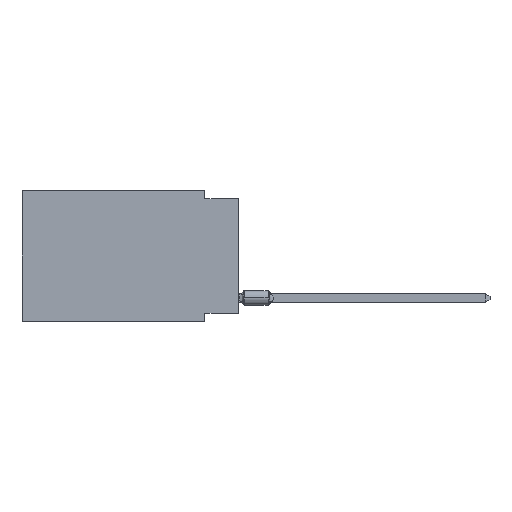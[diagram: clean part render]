
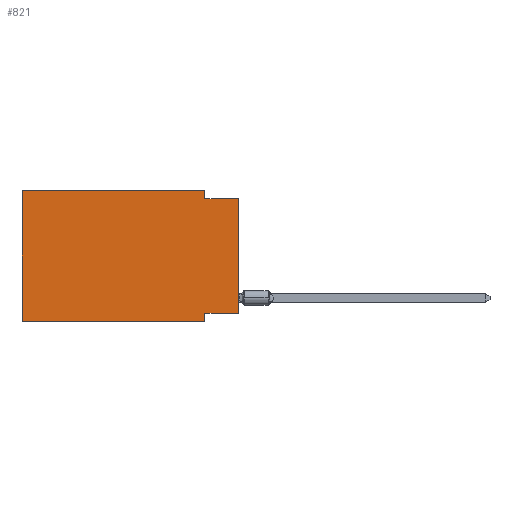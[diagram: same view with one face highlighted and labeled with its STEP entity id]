
A CAD part, left-side view. The second image highlights one B-rep face of the part: STEP entity #821.
In plain terms, the highlighted planar face has unit normal (-1, 0, 0).
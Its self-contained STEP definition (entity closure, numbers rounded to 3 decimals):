
#77 = VECTOR ( 'NONE', #10735, 1000. ) ;
#146 = DIRECTION ( 'NONE',  ( 0., 1., 0. ) ) ;
#390 = CARTESIAN_POINT ( 'NONE',  ( 0., 16.383, 0. ) ) ;
#655 = ORIENTED_EDGE ( 'NONE', *, *, #11525, .T. ) ;
#775 = CARTESIAN_POINT ( 'NONE',  ( 0., 2.54, 0. ) ) ;
#782 = FACE_OUTER_BOUND ( 'NONE', #11068, .T. ) ;
#821 = ADVANCED_FACE ( 'NONE', ( #782 ), #12748, .F. ) ;
#913 = DIRECTION ( 'NONE',  ( 1., 0., 0. ) ) ;
#946 = ORIENTED_EDGE ( 'NONE', *, *, #5960, .F. ) ;
#1041 = DIRECTION ( 'NONE',  ( 0., 0., -1. ) ) ;
#1175 = CARTESIAN_POINT ( 'NONE',  ( 0., 0., -0.635 ) ) ;
#1283 = EDGE_CURVE ( 'NONE', #8576, #7658, #7881, .T. ) ;
#1309 = CARTESIAN_POINT ( 'NONE',  ( 0., 0., -9.271 ) ) ;
#1402 = VECTOR ( 'NONE', #9608, 1000. ) ;
#2330 = CARTESIAN_POINT ( 'NONE',  ( 0., 16.383, -9.906 ) ) ;
#2385 = VECTOR ( 'NONE', #2811, 1000. ) ;
#2516 = VERTEX_POINT ( 'NONE', #5256 ) ;
#2692 = LINE ( 'NONE', #8646, #1402 ) ;
#2745 = CARTESIAN_POINT ( 'NONE',  ( 0., 16.383, 0. ) ) ;
#2811 = DIRECTION ( 'NONE',  ( 0., 0., 1. ) ) ;
#3001 = VECTOR ( 'NONE', #12733, 1000. ) ;
#3041 = ORIENTED_EDGE ( 'NONE', *, *, #8999, .F. ) ;
#3194 = DIRECTION ( 'NONE',  ( 0., -1., 0. ) ) ;
#3314 = VERTEX_POINT ( 'NONE', #2330 ) ;
#3380 = LINE ( 'NONE', #10111, #10528 ) ;
#3882 = CARTESIAN_POINT ( 'NONE',  ( 0., 16.383, 0. ) ) ;
#4348 = LINE ( 'NONE', #8102, #11321 ) ;
#4408 = VECTOR ( 'NONE', #146, 1000. ) ;
#4822 = CARTESIAN_POINT ( 'NONE',  ( 0., 0., -0.635 ) ) ;
#5256 = CARTESIAN_POINT ( 'NONE',  ( 0., 0., -9.271 ) ) ;
#5404 = CARTESIAN_POINT ( 'NONE',  ( 0., 2.54, -9.906 ) ) ;
#5557 = LINE ( 'NONE', #12420, #9496 ) ;
#5960 = EDGE_CURVE ( 'NONE', #3314, #7800, #8635, .T. ) ;
#6137 = LINE ( 'NONE', #1309, #4408 ) ;
#6636 = VERTEX_POINT ( 'NONE', #9379 ) ;
#6744 = EDGE_CURVE ( 'NONE', #7800, #10363, #6772, .T. ) ;
#6772 = LINE ( 'NONE', #9566, #77 ) ;
#6778 = ORIENTED_EDGE ( 'NONE', *, *, #6744, .F. ) ;
#6788 = ORIENTED_EDGE ( 'NONE', *, *, #12698, .T. ) ;
#7200 = CARTESIAN_POINT ( 'NONE',  ( 0., 2.54, -0.635 ) ) ;
#7305 = EDGE_CURVE ( 'NONE', #2516, #6636, #6137, .T. ) ;
#7658 = VERTEX_POINT ( 'NONE', #1175 ) ;
#7800 = VERTEX_POINT ( 'NONE', #390 ) ;
#7881 = LINE ( 'NONE', #4822, #3001 ) ;
#7958 = ORIENTED_EDGE ( 'NONE', *, *, #1283, .F. ) ;
#7971 = ORIENTED_EDGE ( 'NONE', *, *, #12500, .F. ) ;
#8102 = CARTESIAN_POINT ( 'NONE',  ( 0., 0., 0. ) ) ;
#8300 = DIRECTION ( 'NONE',  ( 0., 0., 1. ) ) ;
#8576 = VERTEX_POINT ( 'NONE', #7200 ) ;
#8635 = LINE ( 'NONE', #2745, #2385 ) ;
#8646 = CARTESIAN_POINT ( 'NONE',  ( 0., 2.54, -9.906 ) ) ;
#8999 = EDGE_CURVE ( 'NONE', #10363, #8576, #5557, .T. ) ;
#9379 = CARTESIAN_POINT ( 'NONE',  ( 0., 2.54, -9.271 ) ) ;
#9496 = VECTOR ( 'NONE', #12295, 1000. ) ;
#9503 = VERTEX_POINT ( 'NONE', #5404 ) ;
#9566 = CARTESIAN_POINT ( 'NONE',  ( 0., 16.383, 0. ) ) ;
#9608 = DIRECTION ( 'NONE',  ( 0., 0., -1. ) ) ;
#10111 = CARTESIAN_POINT ( 'NONE',  ( 0., 16.383, -9.906 ) ) ;
#10363 = VERTEX_POINT ( 'NONE', #775 ) ;
#10528 = VECTOR ( 'NONE', #3194, 1000. ) ;
#10735 = DIRECTION ( 'NONE',  ( 0., -1., 0. ) ) ;
#10830 = AXIS2_PLACEMENT_3D ( 'NONE', #3882, #913, #1041 ) ;
#11068 = EDGE_LOOP ( 'NONE', ( #6788, #7958, #3041, #6778, #946, #655, #7971, #12407 ) ) ;
#11321 = VECTOR ( 'NONE', #8300, 1000. ) ;
#11525 = EDGE_CURVE ( 'NONE', #3314, #9503, #3380, .T. ) ;
#12295 = DIRECTION ( 'NONE',  ( 0., 0., -1. ) ) ;
#12407 = ORIENTED_EDGE ( 'NONE', *, *, #7305, .F. ) ;
#12420 = CARTESIAN_POINT ( 'NONE',  ( 0., 2.54, 0. ) ) ;
#12500 = EDGE_CURVE ( 'NONE', #6636, #9503, #2692, .T. ) ;
#12698 = EDGE_CURVE ( 'NONE', #2516, #7658, #4348, .T. ) ;
#12733 = DIRECTION ( 'NONE',  ( 0., -1., 0. ) ) ;
#12748 = PLANE ( 'NONE',  #10830 ) ;
